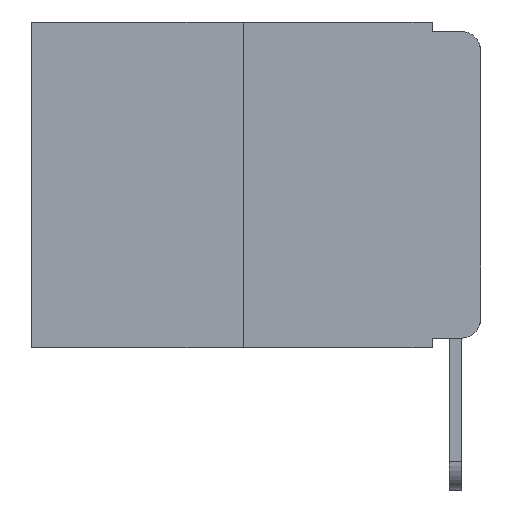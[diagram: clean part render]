
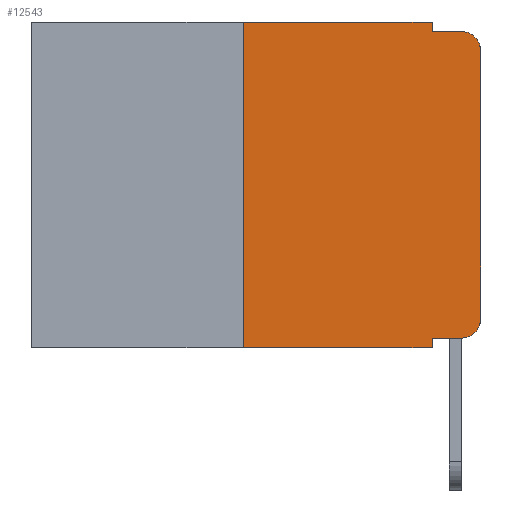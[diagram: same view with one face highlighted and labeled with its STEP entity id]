
A CAD part, left-side view. The second image highlights one B-rep face of the part: STEP entity #12543.
In plain terms, the highlighted planar face has unit normal (-1, 0, 0).
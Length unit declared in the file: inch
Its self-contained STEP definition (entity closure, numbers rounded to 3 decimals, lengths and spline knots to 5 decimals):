
#326 = EDGE_CURVE ( 'NONE', #12074, #8638, #6804, .T. ) ;
#443 = ORIENTED_EDGE ( 'NONE', *, *, #326, .T. ) ;
#535 = DIRECTION ( 'NONE',  ( 0., -1., 0. ) ) ;
#792 = LINE ( 'NONE', #3880, #7585 ) ;
#830 = DIRECTION ( 'NONE',  ( 0., -1., 0. ) ) ;
#859 = DIRECTION ( 'NONE',  ( 0., 0., 1. ) ) ;
#1280 = ORIENTED_EDGE ( 'NONE', *, *, #8827, .F. ) ;
#1534 = CARTESIAN_POINT ( 'NONE',  ( 0., 0.473, -0.343 ) ) ;
#1572 = EDGE_CURVE ( 'NONE', #8320, #12074, #7855, .T. ) ;
#1583 = CARTESIAN_POINT ( 'NONE',  ( 0., 0.02, -0.313 ) ) ;
#1759 = CARTESIAN_POINT ( 'NONE',  ( 0., 0.25, -0.343 ) ) ;
#1790 = ORIENTED_EDGE ( 'NONE', *, *, #1927, .T. ) ;
#1927 = EDGE_CURVE ( 'NONE', #2479, #8320, #6339, .T. ) ;
#1937 = LINE ( 'NONE', #10884, #9442 ) ;
#2222 = VECTOR ( 'NONE', #4666, 39.37008 ) ;
#2349 = CARTESIAN_POINT ( 'NONE',  ( 0., 0.051, 0. ) ) ;
#2440 = EDGE_CURVE ( 'NONE', #7940, #12761, #5567, .T. ) ;
#2479 = VERTEX_POINT ( 'NONE', #4772 ) ;
#2586 = CARTESIAN_POINT ( 'NONE',  ( 0., 0.051, 0. ) ) ;
#2727 = DIRECTION ( 'NONE',  ( 0., 0., -1. ) ) ;
#2734 = DIRECTION ( 'NONE',  ( 0., 0., -1. ) ) ;
#2916 = DIRECTION ( 'NONE',  ( 1., 0., 0. ) ) ;
#2989 = EDGE_CURVE ( 'NONE', #6448, #12546, #1937, .T. ) ;
#3166 = CARTESIAN_POINT ( 'NONE',  ( 0., 0.02, -0.333 ) ) ;
#3352 = EDGE_LOOP ( 'NONE', ( #443, #9258, #4717, #6192, #7187, #12688, #8014, #1280, #1790, #9622 ) ) ;
#3462 = AXIS2_PLACEMENT_3D ( 'NONE', #12741, #3610, #11731 ) ;
#3610 = DIRECTION ( 'NONE',  ( -1., 0., 0. ) ) ;
#3678 = CARTESIAN_POINT ( 'NONE',  ( 0., 0., -0.313 ) ) ;
#3811 = VECTOR ( 'NONE', #12647, 39.37008 ) ;
#3880 = CARTESIAN_POINT ( 'NONE',  ( 0., 0.051, 0. ) ) ;
#4078 = VERTEX_POINT ( 'NONE', #2349 ) ;
#4553 = VECTOR ( 'NONE', #2727, 39.37008 ) ;
#4565 = VECTOR ( 'NONE', #6538, 39.37008 ) ;
#4666 = DIRECTION ( 'NONE',  ( 0., 0., 1. ) ) ;
#4717 = ORIENTED_EDGE ( 'NONE', *, *, #2440, .F. ) ;
#4772 = CARTESIAN_POINT ( 'NONE',  ( 0., 0.051, -0.333 ) ) ;
#4949 = VERTEX_POINT ( 'NONE', #12638 ) ;
#5110 = CARTESIAN_POINT ( 'NONE',  ( 0., 0.473, 0. ) ) ;
#5386 = CIRCLE ( 'NONE', #3462, 0.02 ) ;
#5567 = LINE ( 'NONE', #10834, #3811 ) ;
#5617 = VECTOR ( 'NONE', #830, 39.37008 ) ;
#5622 = CARTESIAN_POINT ( 'NONE',  ( 0., 0., -0.03 ) ) ;
#5795 = CARTESIAN_POINT ( 'NONE',  ( 0., 0., 0. ) ) ;
#5909 = EDGE_CURVE ( 'NONE', #4078, #7940, #10729, .T. ) ;
#6043 = VECTOR ( 'NONE', #535, 39.37008 ) ;
#6192 = ORIENTED_EDGE ( 'NONE', *, *, #5909, .F. ) ;
#6339 = LINE ( 'NONE', #7408, #4565 ) ;
#6448 = VERTEX_POINT ( 'NONE', #1759 ) ;
#6538 = DIRECTION ( 'NONE',  ( 0., -1., 0. ) ) ;
#6766 = LINE ( 'NONE', #1534, #6043 ) ;
#6804 = LINE ( 'NONE', #5795, #2222 ) ;
#6993 = FACE_OUTER_BOUND ( 'NONE', #3352, .T. ) ;
#7124 = CARTESIAN_POINT ( 'NONE',  ( 0., 0.051, -0.01 ) ) ;
#7187 = ORIENTED_EDGE ( 'NONE', *, *, #10909, .F. ) ;
#7408 = CARTESIAN_POINT ( 'NONE',  ( 0., 0.051, -0.333 ) ) ;
#7585 = VECTOR ( 'NONE', #11145, 39.37008 ) ;
#7785 = PLANE ( 'NONE',  #11619 ) ;
#7855 = CIRCLE ( 'NONE', #11253, 0.02 ) ;
#7940 = VERTEX_POINT ( 'NONE', #7124 ) ;
#8014 = ORIENTED_EDGE ( 'NONE', *, *, #10036, .T. ) ;
#8123 = LINE ( 'NONE', #5110, #5617 ) ;
#8320 = VERTEX_POINT ( 'NONE', #3166 ) ;
#8638 = VERTEX_POINT ( 'NONE', #5622 ) ;
#8827 = EDGE_CURVE ( 'NONE', #2479, #4949, #792, .T. ) ;
#9258 = ORIENTED_EDGE ( 'NONE', *, *, #10442, .T. ) ;
#9442 = VECTOR ( 'NONE', #859, 39.37008 ) ;
#9622 = ORIENTED_EDGE ( 'NONE', *, *, #1572, .T. ) ;
#9736 = DIRECTION ( 'NONE',  ( -1., 0., 0. ) ) ;
#10036 = EDGE_CURVE ( 'NONE', #6448, #4949, #6766, .T. ) ;
#10105 = DIRECTION ( 'NONE',  ( 0., 0., -1. ) ) ;
#10442 = EDGE_CURVE ( 'NONE', #8638, #12761, #5386, .T. ) ;
#10635 = CARTESIAN_POINT ( 'NONE',  ( 0., 0.02, -0.01 ) ) ;
#10729 = LINE ( 'NONE', #2586, #4553 ) ;
#10834 = CARTESIAN_POINT ( 'NONE',  ( 0., 0.051, -0.01 ) ) ;
#10884 = CARTESIAN_POINT ( 'NONE',  ( 0., 0.25, 0. ) ) ;
#10907 = CARTESIAN_POINT ( 'NONE',  ( 0., 0.473, 0. ) ) ;
#10909 = EDGE_CURVE ( 'NONE', #12546, #4078, #8123, .T. ) ;
#11145 = DIRECTION ( 'NONE',  ( 0., 0., -1. ) ) ;
#11253 = AXIS2_PLACEMENT_3D ( 'NONE', #1583, #9736, #2734 ) ;
#11619 = AXIS2_PLACEMENT_3D ( 'NONE', #10907, #2916, #10105 ) ;
#11731 = DIRECTION ( 'NONE',  ( 0., 0., -1. ) ) ;
#12074 = VERTEX_POINT ( 'NONE', #3678 ) ;
#12543 = ADVANCED_FACE ( 'NONE', ( #6993 ), #7785, .F. ) ;
#12546 = VERTEX_POINT ( 'NONE', #13113 ) ;
#12638 = CARTESIAN_POINT ( 'NONE',  ( 0., 0.051, -0.343 ) ) ;
#12647 = DIRECTION ( 'NONE',  ( 0., -1., 0. ) ) ;
#12688 = ORIENTED_EDGE ( 'NONE', *, *, #2989, .F. ) ;
#12741 = CARTESIAN_POINT ( 'NONE',  ( 0., 0.02, -0.03 ) ) ;
#12761 = VERTEX_POINT ( 'NONE', #10635 ) ;
#13113 = CARTESIAN_POINT ( 'NONE',  ( 0., 0.25, 0. ) ) ;
